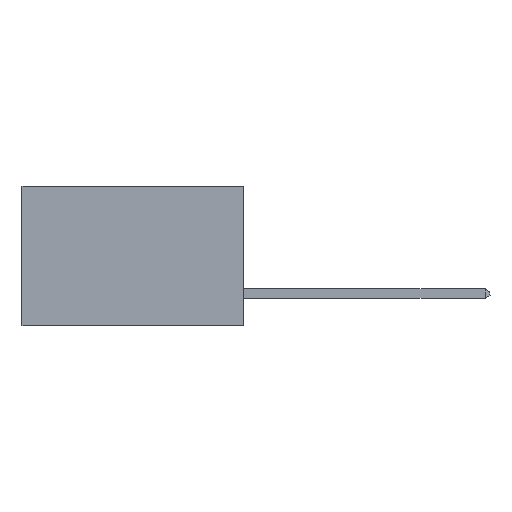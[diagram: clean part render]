
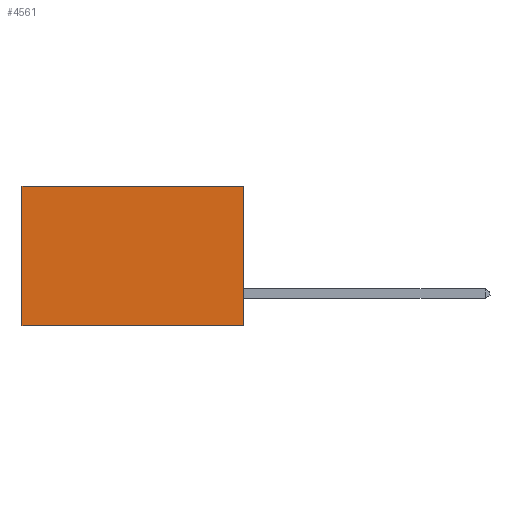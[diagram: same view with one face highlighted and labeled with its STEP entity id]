
A CAD part, left-side view. The second image highlights one B-rep face of the part: STEP entity #4561.
In plain terms, the highlighted planar face has unit normal (-1, 0, 0).
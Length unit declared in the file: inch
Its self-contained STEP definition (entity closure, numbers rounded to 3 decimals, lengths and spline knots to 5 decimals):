
#201 = EDGE_CURVE ( 'NONE', #6232, #224, #5218, .T. ) ;
#221 = CARTESIAN_POINT ( 'NONE',  ( 0.277, 0.59, 0. ) ) ;
#224 = VERTEX_POINT ( 'NONE', #10307 ) ;
#370 = DIRECTION ( 'NONE',  ( 1., 0., 0. ) ) ;
#887 = LINE ( 'NONE', #2379, #8796 ) ;
#1265 = DIRECTION ( 'NONE',  ( 0., 1., 0. ) ) ;
#1881 = LINE ( 'NONE', #11787, #7929 ) ;
#2161 = EDGE_CURVE ( 'NONE', #224, #4201, #3460, .T. ) ;
#2284 = DIRECTION ( 'NONE',  ( 0., 0., -1. ) ) ;
#2379 = CARTESIAN_POINT ( 'NONE',  ( 0.277, 0.59, -0.37 ) ) ;
#2698 = EDGE_LOOP ( 'NONE', ( #12631, #12649, #12413, #8909 ) ) ;
#3007 = EDGE_CURVE ( 'NONE', #6232, #6397, #1881, .T. ) ;
#3282 = FACE_OUTER_BOUND ( 'NONE', #2698, .T. ) ;
#3336 = CARTESIAN_POINT ( 'NONE',  ( 0.277, 0., -0.37 ) ) ;
#3337 = CARTESIAN_POINT ( 'NONE',  ( 0.277, 0., 0. ) ) ;
#3460 = LINE ( 'NONE', #13510, #3807 ) ;
#3807 = VECTOR ( 'NONE', #1265, 39.37008 ) ;
#4054 = CARTESIAN_POINT ( 'NONE',  ( 0.277, 0.59, -0.37 ) ) ;
#4201 = VERTEX_POINT ( 'NONE', #4054 ) ;
#4350 = CARTESIAN_POINT ( 'NONE',  ( 0.277, 0., -0.37 ) ) ;
#4561 = ADVANCED_FACE ( 'NONE', ( #3282 ), #13139, .F. ) ;
#5218 = LINE ( 'NONE', #4350, #13036 ) ;
#5516 = DIRECTION ( 'NONE',  ( 0., 1., 0. ) ) ;
#5835 = DIRECTION ( 'NONE',  ( 0., 0., -1. ) ) ;
#5895 = AXIS2_PLACEMENT_3D ( 'NONE', #3336, #370, #2284 ) ;
#6232 = VERTEX_POINT ( 'NONE', #3337 ) ;
#6397 = VERTEX_POINT ( 'NONE', #221 ) ;
#7929 = VECTOR ( 'NONE', #5516, 39.37008 ) ;
#8748 = DIRECTION ( 'NONE',  ( 0., 0., -1. ) ) ;
#8796 = VECTOR ( 'NONE', #8748, 39.37008 ) ;
#8909 = ORIENTED_EDGE ( 'NONE', *, *, #3007, .T. ) ;
#10307 = CARTESIAN_POINT ( 'NONE',  ( 0.277, 0., -0.37 ) ) ;
#11787 = CARTESIAN_POINT ( 'NONE',  ( 0.277, 0., 0. ) ) ;
#12129 = EDGE_CURVE ( 'NONE', #6397, #4201, #887, .T. ) ;
#12413 = ORIENTED_EDGE ( 'NONE', *, *, #201, .F. ) ;
#12631 = ORIENTED_EDGE ( 'NONE', *, *, #12129, .T. ) ;
#12649 = ORIENTED_EDGE ( 'NONE', *, *, #2161, .F. ) ;
#13036 = VECTOR ( 'NONE', #5835, 39.37008 ) ;
#13139 = PLANE ( 'NONE',  #5895 ) ;
#13510 = CARTESIAN_POINT ( 'NONE',  ( 0.277, 0., -0.37 ) ) ;
